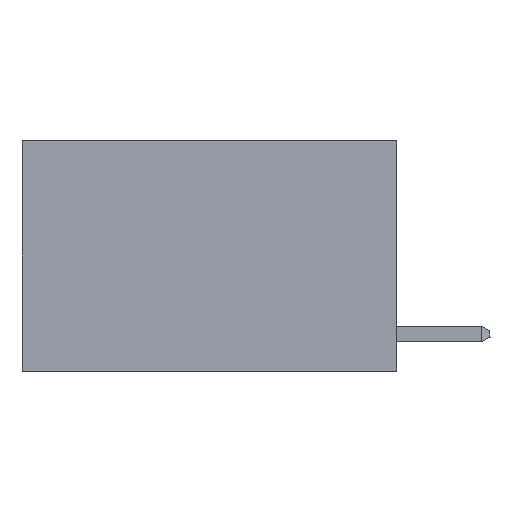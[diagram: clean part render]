
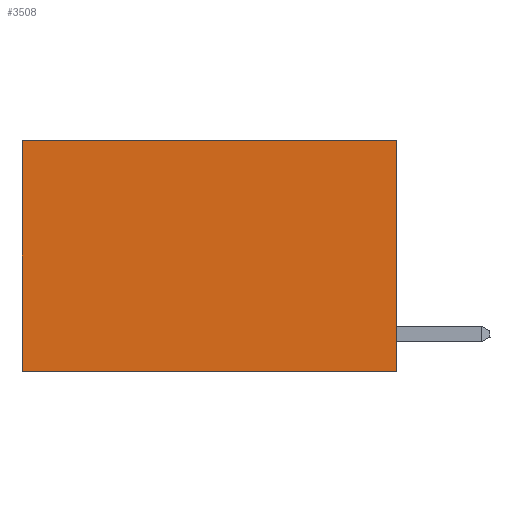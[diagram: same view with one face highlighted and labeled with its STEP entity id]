
A CAD part, left-side view. The second image highlights one B-rep face of the part: STEP entity #3508.
In plain terms, the highlighted planar face has unit normal (-1, 0, 0).
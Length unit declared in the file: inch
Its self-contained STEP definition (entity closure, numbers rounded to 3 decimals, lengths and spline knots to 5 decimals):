
#684 = VECTOR ( 'NONE', #11859, 39.37008 ) ;
#814 = CARTESIAN_POINT ( 'NONE',  ( 0.2625, 0.6, 0. ) ) ;
#1224 = EDGE_CURVE ( 'NONE', #16443, #2201, #16062, .T. ) ;
#1336 = DIRECTION ( 'NONE',  ( 1., 0., 0. ) ) ;
#1699 = DIRECTION ( 'NONE',  ( 0., 0., -1. ) ) ;
#2201 = VERTEX_POINT ( 'NONE', #17143 ) ;
#2570 = LINE ( 'NONE', #14830, #684 ) ;
#2712 = PLANE ( 'NONE',  #15448 ) ;
#3508 = ADVANCED_FACE ( 'NONE', ( #10730 ), #2712, .F. ) ;
#3645 = CARTESIAN_POINT ( 'NONE',  ( 0.2625, 0., 0. ) ) ;
#5330 = ORIENTED_EDGE ( 'NONE', *, *, #13301, .F. ) ;
#6365 = ORIENTED_EDGE ( 'NONE', *, *, #16010, .T. ) ;
#6744 = CARTESIAN_POINT ( 'NONE',  ( 0.2625, 0., -0.37 ) ) ;
#7649 = CARTESIAN_POINT ( 'NONE',  ( 0.2625, 0., 0. ) ) ;
#8005 = VECTOR ( 'NONE', #1699, 39.37008 ) ;
#8262 = DIRECTION ( 'NONE',  ( 0., 1., 0. ) ) ;
#8469 = LINE ( 'NONE', #7649, #8005 ) ;
#8738 = VECTOR ( 'NONE', #15297, 39.37008 ) ;
#9226 = ORIENTED_EDGE ( 'NONE', *, *, #1224, .T. ) ;
#10387 = EDGE_CURVE ( 'NONE', #11325, #15817, #8469, .T. ) ;
#10566 = EDGE_LOOP ( 'NONE', ( #9226, #5330, #15287, #6365 ) ) ;
#10730 = FACE_OUTER_BOUND ( 'NONE', #10566, .T. ) ;
#11325 = VERTEX_POINT ( 'NONE', #3645 ) ;
#11508 = CARTESIAN_POINT ( 'NONE',  ( 0.2625, 0., -0.37 ) ) ;
#11859 = DIRECTION ( 'NONE',  ( 0., 1., 0. ) ) ;
#13204 = CARTESIAN_POINT ( 'NONE',  ( 0.2625, 0., 0. ) ) ;
#13301 = EDGE_CURVE ( 'NONE', #15817, #2201, #17523, .T. ) ;
#14530 = CARTESIAN_POINT ( 'NONE',  ( 0.2625, 0.6, 0. ) ) ;
#14830 = CARTESIAN_POINT ( 'NONE',  ( 0.2625, 0., 0. ) ) ;
#15287 = ORIENTED_EDGE ( 'NONE', *, *, #10387, .F. ) ;
#15297 = DIRECTION ( 'NONE',  ( 0., 0., -1. ) ) ;
#15448 = AXIS2_PLACEMENT_3D ( 'NONE', #13204, #1336, #17588 ) ;
#15817 = VERTEX_POINT ( 'NONE', #11508 ) ;
#16010 = EDGE_CURVE ( 'NONE', #11325, #16443, #2570, .T. ) ;
#16062 = LINE ( 'NONE', #14530, #8738 ) ;
#16443 = VERTEX_POINT ( 'NONE', #814 ) ;
#16573 = VECTOR ( 'NONE', #8262, 39.37008 ) ;
#17143 = CARTESIAN_POINT ( 'NONE',  ( 0.2625, 0.6, -0.37 ) ) ;
#17523 = LINE ( 'NONE', #6744, #16573 ) ;
#17588 = DIRECTION ( 'NONE',  ( 0., 0., -1. ) ) ;
